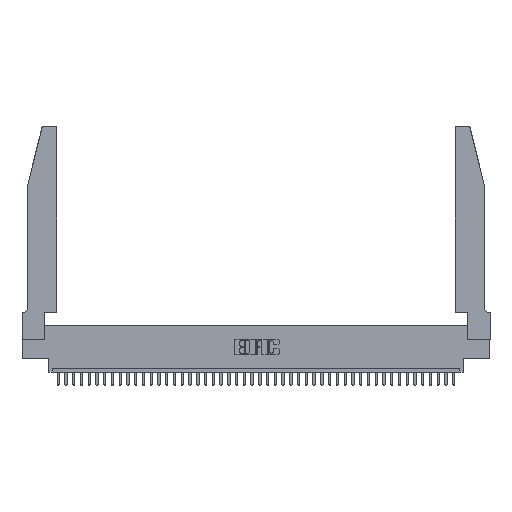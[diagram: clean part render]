
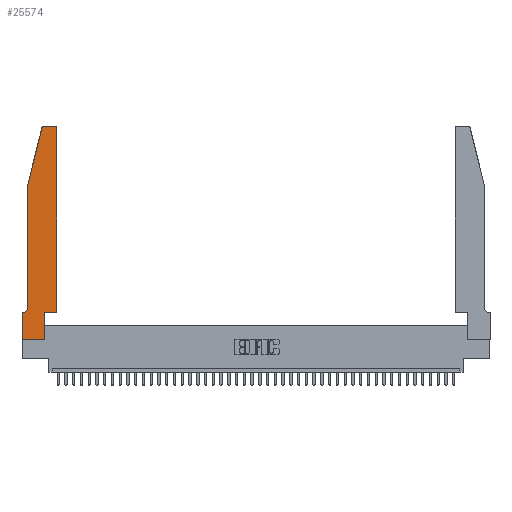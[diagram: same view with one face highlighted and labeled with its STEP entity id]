
A CAD part, top view. The second image highlights one B-rep face of the part: STEP entity #25574.
In plain terms, the highlighted planar face has unit normal (0, 0, 1).
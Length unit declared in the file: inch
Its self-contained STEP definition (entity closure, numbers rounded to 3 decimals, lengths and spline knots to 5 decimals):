
#339 = ORIENTED_EDGE ( 'NONE', *, *, #22784, .T. ) ;
#1807 = DIRECTION ( 'NONE',  ( 1., 0., 0. ) ) ;
#2507 = LINE ( 'NONE', #10997, #10733 ) ;
#2755 = DIRECTION ( 'NONE',  ( -0.239, -0.971, 0. ) ) ;
#3595 = LINE ( 'NONE', #34215, #33006 ) ;
#3974 = CARTESIAN_POINT ( 'NONE',  ( 0., 0.35, 0.37 ) ) ;
#3980 = CARTESIAN_POINT ( 'NONE',  ( 0., 0., 0.37 ) ) ;
#4104 = LINE ( 'NONE', #39534, #20583 ) ;
#4899 = LINE ( 'NONE', #29644, #42097 ) ;
#5794 = EDGE_CURVE ( 'NONE', #37746, #21221, #10331, .T. ) ;
#5850 = FACE_OUTER_BOUND ( 'NONE', #26860, .T. ) ;
#6020 = CARTESIAN_POINT ( 'NONE',  ( 0., 0., 0.37 ) ) ;
#6064 = VERTEX_POINT ( 'NONE', #12895 ) ;
#6447 = DIRECTION ( 'NONE',  ( -1., 0., 0. ) ) ;
#9005 = VERTEX_POINT ( 'NONE', #6020 ) ;
#9803 = EDGE_CURVE ( 'NONE', #21221, #36338, #3595, .T. ) ;
#9934 = CIRCLE ( 'NONE', #19324, 0.03 ) ;
#10227 = ORIENTED_EDGE ( 'NONE', *, *, #38081, .T. ) ;
#10331 = LINE ( 'NONE', #16809, #20144 ) ;
#10684 = VERTEX_POINT ( 'NONE', #25925 ) ;
#10733 = VECTOR ( 'NONE', #40904, 39.37008 ) ;
#10997 = CARTESIAN_POINT ( 'NONE',  ( 0.4505, 0.35, 0.37 ) ) ;
#11000 = DIRECTION ( 'NONE',  ( 1., 0., 0. ) ) ;
#11153 = CARTESIAN_POINT ( 'NONE',  ( 0.4205, 2.72, 0.37 ) ) ;
#11522 = VERTEX_POINT ( 'NONE', #24788 ) ;
#12741 = AXIS2_PLACEMENT_3D ( 'NONE', #3974, #36694, #20228 ) ;
#12895 = CARTESIAN_POINT ( 'NONE',  ( 0., 0.35, 0.37 ) ) ;
#13036 = EDGE_CURVE ( 'NONE', #13994, #38397, #4104, .T. ) ;
#13528 = CARTESIAN_POINT ( 'NONE',  ( 0.0755, 0.35, 0.37 ) ) ;
#13994 = VERTEX_POINT ( 'NONE', #35263 ) ;
#14688 = CARTESIAN_POINT ( 'NONE',  ( 0.2865, 0.35, 0.37 ) ) ;
#15176 = VERTEX_POINT ( 'NONE', #33268 ) ;
#15804 = CIRCLE ( 'NONE', #33031, 0.03 ) ;
#15875 = VECTOR ( 'NONE', #30910, 39.37008 ) ;
#15921 = DIRECTION ( 'NONE',  ( 1., 0., 0. ) ) ;
#16798 = ORIENTED_EDGE ( 'NONE', *, *, #29348, .T. ) ;
#16809 = CARTESIAN_POINT ( 'NONE',  ( 0.2865, 0.35, 0.37 ) ) ;
#17564 = ORIENTED_EDGE ( 'NONE', *, *, #13036, .T. ) ;
#18234 = DIRECTION ( 'NONE',  ( -1., 0., 0. ) ) ;
#18387 = EDGE_CURVE ( 'NONE', #11522, #13994, #15804, .T. ) ;
#19324 = AXIS2_PLACEMENT_3D ( 'NONE', #11153, #21563, #1807 ) ;
#19489 = LINE ( 'NONE', #13528, #40166 ) ;
#19667 = DIRECTION ( 'NONE',  ( 0., -1., 0. ) ) ;
#20144 = VECTOR ( 'NONE', #23187, 39.37008 ) ;
#20228 = DIRECTION ( 'NONE',  ( 1., 0., 0. ) ) ;
#20583 = VECTOR ( 'NONE', #2755, 39.37008 ) ;
#20963 = AXIS2_PLACEMENT_3D ( 'NONE', #38056, #24469, #18234 ) ;
#21221 = VERTEX_POINT ( 'NONE', #14688 ) ;
#21312 = ORIENTED_EDGE ( 'NONE', *, *, #26393, .T. ) ;
#21563 = DIRECTION ( 'NONE',  ( 0., 0., 1. ) ) ;
#22271 = DIRECTION ( 'NONE',  ( 0., 0., 1. ) ) ;
#22491 = LINE ( 'NONE', #35150, #24556 ) ;
#22592 = LINE ( 'NONE', #33772, #15875 ) ;
#22784 = EDGE_CURVE ( 'NONE', #6064, #9005, #22592, .T. ) ;
#23078 = ORIENTED_EDGE ( 'NONE', *, *, #9803, .T. ) ;
#23187 = DIRECTION ( 'NONE',  ( 0., 1., 0. ) ) ;
#24469 = DIRECTION ( 'NONE',  ( 0., 0., -1. ) ) ;
#24556 = VECTOR ( 'NONE', #6447, 39.37008 ) ;
#24788 = CARTESIAN_POINT ( 'NONE',  ( 0.284, 2.75, 0.37 ) ) ;
#25468 = CARTESIAN_POINT ( 'NONE',  ( 0.0055, 0.35, 0.37 ) ) ;
#25574 = ADVANCED_FACE ( 'NONE', ( #5850 ), #26749, .T. ) ;
#25925 = CARTESIAN_POINT ( 'NONE',  ( 0.4205, 2.75, 0.37 ) ) ;
#26079 = ORIENTED_EDGE ( 'NONE', *, *, #40035, .T. ) ;
#26393 = EDGE_CURVE ( 'NONE', #27163, #6064, #19489, .T. ) ;
#26749 = PLANE ( 'NONE',  #12741 ) ;
#26860 = EDGE_LOOP ( 'NONE', ( #10227, #40895, #17564, #39381, #16798, #21312, #339, #37048, #33835, #23078, #33242, #26079 ) ) ;
#27040 = CIRCLE ( 'NONE', #20963, 0.07 ) ;
#27116 = CARTESIAN_POINT ( 'NONE',  ( 0.2865, 0., 0.37 ) ) ;
#27163 = VERTEX_POINT ( 'NONE', #25468 ) ;
#27493 = EDGE_CURVE ( 'NONE', #9005, #37746, #34355, .T. ) ;
#27848 = EDGE_CURVE ( 'NONE', #38397, #29923, #4899, .T. ) ;
#28040 = CARTESIAN_POINT ( 'NONE',  ( 0.0755, 0.42, 0.37 ) ) ;
#29183 = VECTOR ( 'NONE', #11000, 39.37008 ) ;
#29348 = EDGE_CURVE ( 'NONE', #29923, #27163, #27040, .T. ) ;
#29644 = CARTESIAN_POINT ( 'NONE',  ( 0.0755, 2., 0.37 ) ) ;
#29923 = VERTEX_POINT ( 'NONE', #28040 ) ;
#30910 = DIRECTION ( 'NONE',  ( 0., -1., 0. ) ) ;
#31670 = CARTESIAN_POINT ( 'NONE',  ( 0.0755, 2., 0.37 ) ) ;
#33006 = VECTOR ( 'NONE', #40873, 39.37008 ) ;
#33031 = AXIS2_PLACEMENT_3D ( 'NONE', #42241, #22271, #15921 ) ;
#33242 = ORIENTED_EDGE ( 'NONE', *, *, #42426, .T. ) ;
#33268 = CARTESIAN_POINT ( 'NONE',  ( 0.4505, 2.72, 0.37 ) ) ;
#33749 = DIRECTION ( 'NONE',  ( -1., 0., 0. ) ) ;
#33772 = CARTESIAN_POINT ( 'NONE',  ( 0., 0., 0.37 ) ) ;
#33835 = ORIENTED_EDGE ( 'NONE', *, *, #5794, .T. ) ;
#34215 = CARTESIAN_POINT ( 'NONE',  ( 0.4505, 0.35, 0.37 ) ) ;
#34355 = LINE ( 'NONE', #3980, #29183 ) ;
#35150 = CARTESIAN_POINT ( 'NONE',  ( 0.2605, 2.75, 0.37 ) ) ;
#35263 = CARTESIAN_POINT ( 'NONE',  ( 0.25487, 2.72718, 0.37 ) ) ;
#36290 = CARTESIAN_POINT ( 'NONE',  ( 0.4505, 0.35, 0.37 ) ) ;
#36338 = VERTEX_POINT ( 'NONE', #36290 ) ;
#36694 = DIRECTION ( 'NONE',  ( 0., 0., 1. ) ) ;
#37048 = ORIENTED_EDGE ( 'NONE', *, *, #27493, .T. ) ;
#37746 = VERTEX_POINT ( 'NONE', #27116 ) ;
#38056 = CARTESIAN_POINT ( 'NONE',  ( 0.0055, 0.42, 0.37 ) ) ;
#38081 = EDGE_CURVE ( 'NONE', #10684, #11522, #22491, .T. ) ;
#38397 = VERTEX_POINT ( 'NONE', #31670 ) ;
#39381 = ORIENTED_EDGE ( 'NONE', *, *, #27848, .T. ) ;
#39534 = CARTESIAN_POINT ( 'NONE',  ( 0.0755, 2., 0.37 ) ) ;
#40035 = EDGE_CURVE ( 'NONE', #15176, #10684, #9934, .T. ) ;
#40166 = VECTOR ( 'NONE', #33749, 39.37008 ) ;
#40873 = DIRECTION ( 'NONE',  ( 1., 0., 0. ) ) ;
#40895 = ORIENTED_EDGE ( 'NONE', *, *, #18387, .T. ) ;
#40904 = DIRECTION ( 'NONE',  ( 0., 1., 0. ) ) ;
#42097 = VECTOR ( 'NONE', #19667, 39.37008 ) ;
#42241 = CARTESIAN_POINT ( 'NONE',  ( 0.284, 2.72, 0.37 ) ) ;
#42426 = EDGE_CURVE ( 'NONE', #36338, #15176, #2507, .T. ) ;
